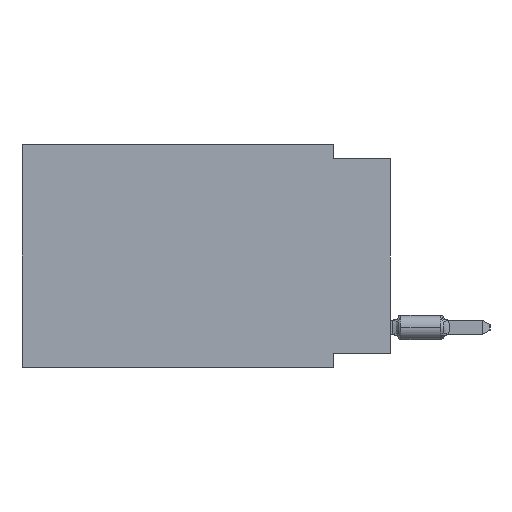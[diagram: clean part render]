
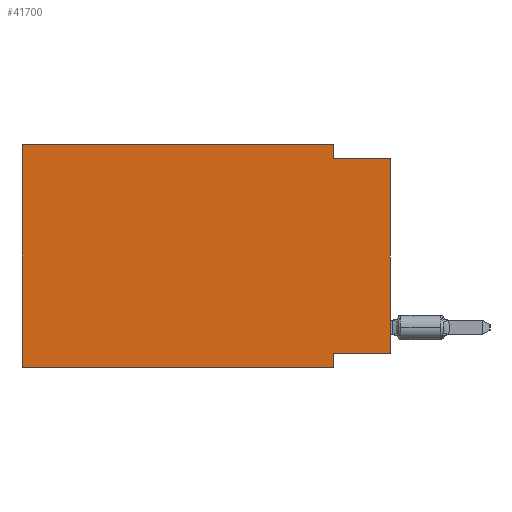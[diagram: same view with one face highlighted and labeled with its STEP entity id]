
A CAD part, left-side view. The second image highlights one B-rep face of the part: STEP entity #41700.
In plain terms, the highlighted planar face has unit normal (-1, 0, 0).
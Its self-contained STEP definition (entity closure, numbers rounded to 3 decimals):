
#918 = VECTOR ( 'NONE', #2718, 1000. ) ;
#1814 = DIRECTION ( 'NONE',  ( 0., 0., -1. ) ) ;
#2718 = DIRECTION ( 'NONE',  ( 0., -1., 0. ) ) ;
#2802 = DIRECTION ( 'NONE',  ( 0., -1., 0. ) ) ;
#3605 = LINE ( 'NONE', #43283, #18911 ) ;
#4495 = CARTESIAN_POINT ( 'NONE',  ( 0., 2.54, -9.271 ) ) ;
#5704 = LINE ( 'NONE', #38242, #57431 ) ;
#6753 = VERTEX_POINT ( 'NONE', #53652 ) ;
#7369 = CARTESIAN_POINT ( 'NONE',  ( 0., 16.383, 0. ) ) ;
#9010 = VERTEX_POINT ( 'NONE', #47070 ) ;
#9017 = VECTOR ( 'NONE', #2802, 1000. ) ;
#9884 = CARTESIAN_POINT ( 'NONE',  ( 0., 16.383, -9.906 ) ) ;
#11440 = DIRECTION ( 'NONE',  ( 0., 1., 0. ) ) ;
#13986 = CARTESIAN_POINT ( 'NONE',  ( 0., 16.383, 0. ) ) ;
#17296 = CARTESIAN_POINT ( 'NONE',  ( 0., 16.383, -9.906 ) ) ;
#18911 = VECTOR ( 'NONE', #51740, 1000. ) ;
#20661 = LINE ( 'NONE', #13986, #26589 ) ;
#21037 = VECTOR ( 'NONE', #36841, 1000. ) ;
#23172 = CARTESIAN_POINT ( 'NONE',  ( 0., 0., -0.635 ) ) ;
#23250 = EDGE_CURVE ( 'NONE', #50159, #6753, #3605, .T. ) ;
#25100 = VECTOR ( 'NONE', #1814, 1000. ) ;
#25655 = DIRECTION ( 'NONE',  ( 1., 0., 0. ) ) ;
#26071 = CARTESIAN_POINT ( 'NONE',  ( 0., 16.383, 0. ) ) ;
#26589 = VECTOR ( 'NONE', #68361, 1000. ) ;
#27257 = ORIENTED_EDGE ( 'NONE', *, *, #23250, .F. ) ;
#28668 = VERTEX_POINT ( 'NONE', #4495 ) ;
#29755 = CARTESIAN_POINT ( 'NONE',  ( 0., 2.54, -9.906 ) ) ;
#31029 = CARTESIAN_POINT ( 'NONE',  ( 0., 16.383, 0. ) ) ;
#31473 = CARTESIAN_POINT ( 'NONE',  ( 0., 0., -0.635 ) ) ;
#31881 = EDGE_LOOP ( 'NONE', ( #84993, #42170, #27257, #84701, #66954, #64935, #38525, #52574 ) ) ;
#35126 = VERTEX_POINT ( 'NONE', #31473 ) ;
#35353 = VERTEX_POINT ( 'NONE', #7369 ) ;
#36240 = VERTEX_POINT ( 'NONE', #17296 ) ;
#36841 = DIRECTION ( 'NONE',  ( 0., -1., 0. ) ) ;
#37815 = VECTOR ( 'NONE', #11440, 1000. ) ;
#38242 = CARTESIAN_POINT ( 'NONE',  ( 0., 0., 0. ) ) ;
#38525 = ORIENTED_EDGE ( 'NONE', *, *, #49328, .F. ) ;
#41700 = ADVANCED_FACE ( 'NONE', ( #65767 ), #58650, .F. ) ;
#42170 = ORIENTED_EDGE ( 'NONE', *, *, #82849, .F. ) ;
#42881 = LINE ( 'NONE', #9884, #9017 ) ;
#43283 = CARTESIAN_POINT ( 'NONE',  ( 0., 2.54, 0. ) ) ;
#46769 = AXIS2_PLACEMENT_3D ( 'NONE', #26071, #25655, #59985 ) ;
#47070 = CARTESIAN_POINT ( 'NONE',  ( 0., 0., -9.271 ) ) ;
#49328 = EDGE_CURVE ( 'NONE', #28668, #74973, #56635, .T. ) ;
#49928 = CARTESIAN_POINT ( 'NONE',  ( 0., 2.54, -9.906 ) ) ;
#50159 = VERTEX_POINT ( 'NONE', #68046 ) ;
#50219 = LINE ( 'NONE', #31029, #21037 ) ;
#51740 = DIRECTION ( 'NONE',  ( 0., 0., -1. ) ) ;
#52060 = DIRECTION ( 'NONE',  ( 0., 0., 1. ) ) ;
#52574 = ORIENTED_EDGE ( 'NONE', *, *, #74997, .F. ) ;
#53652 = CARTESIAN_POINT ( 'NONE',  ( 0., 2.54, -0.635 ) ) ;
#54299 = EDGE_CURVE ( 'NONE', #9010, #35126, #5704, .T. ) ;
#56635 = LINE ( 'NONE', #49928, #25100 ) ;
#57431 = VECTOR ( 'NONE', #52060, 1000. ) ;
#58650 = PLANE ( 'NONE',  #46769 ) ;
#59985 = DIRECTION ( 'NONE',  ( 0., 0., -1. ) ) ;
#60842 = EDGE_CURVE ( 'NONE', #35353, #50159, #50219, .T. ) ;
#64935 = ORIENTED_EDGE ( 'NONE', *, *, #70257, .T. ) ;
#65767 = FACE_OUTER_BOUND ( 'NONE', #31881, .T. ) ;
#66954 = ORIENTED_EDGE ( 'NONE', *, *, #75656, .F. ) ;
#68046 = CARTESIAN_POINT ( 'NONE',  ( 0., 2.54, 0. ) ) ;
#68361 = DIRECTION ( 'NONE',  ( 0., 0., 1. ) ) ;
#70257 = EDGE_CURVE ( 'NONE', #36240, #74973, #42881, .T. ) ;
#71202 = LINE ( 'NONE', #77886, #37815 ) ;
#74973 = VERTEX_POINT ( 'NONE', #29755 ) ;
#74997 = EDGE_CURVE ( 'NONE', #9010, #28668, #71202, .T. ) ;
#75656 = EDGE_CURVE ( 'NONE', #36240, #35353, #20661, .T. ) ;
#76240 = LINE ( 'NONE', #23172, #918 ) ;
#77886 = CARTESIAN_POINT ( 'NONE',  ( 0., 0., -9.271 ) ) ;
#82849 = EDGE_CURVE ( 'NONE', #6753, #35126, #76240, .T. ) ;
#84701 = ORIENTED_EDGE ( 'NONE', *, *, #60842, .F. ) ;
#84993 = ORIENTED_EDGE ( 'NONE', *, *, #54299, .T. ) ;
